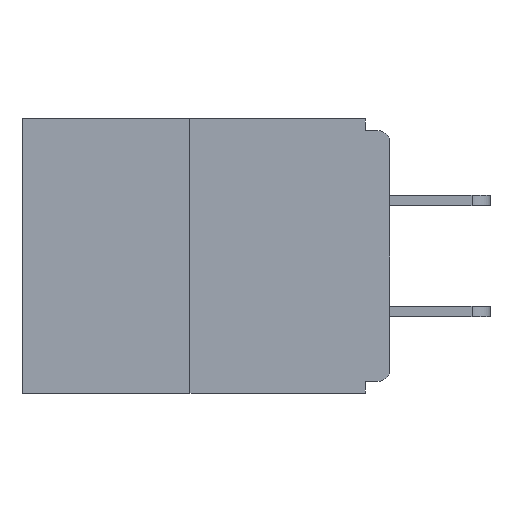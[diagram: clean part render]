
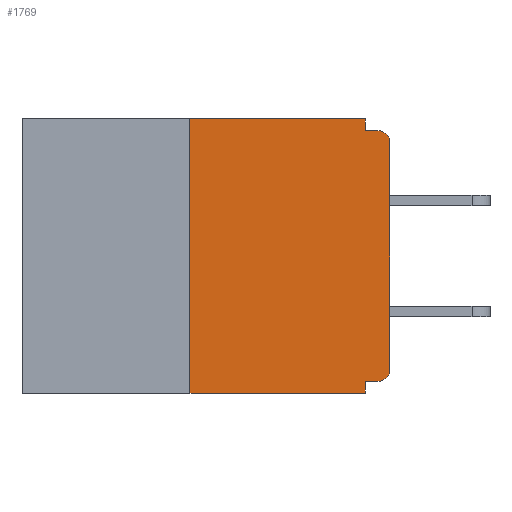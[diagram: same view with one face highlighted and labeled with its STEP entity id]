
A CAD part, left-side view. The second image highlights one B-rep face of the part: STEP entity #1769.
In plain terms, the highlighted planar face has unit normal (-1, 0, 0).
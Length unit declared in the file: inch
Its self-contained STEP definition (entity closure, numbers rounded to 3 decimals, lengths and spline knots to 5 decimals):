
#160 = DIRECTION ( 'NONE',  ( 0., 0., 1. ) ) ;
#436 = VECTOR ( 'NONE', #3665, 39.37008 ) ;
#724 = LINE ( 'NONE', #1875, #4259 ) ;
#869 = AXIS2_PLACEMENT_3D ( 'NONE', #11613, #14555, #8751 ) ;
#894 = CARTESIAN_POINT ( 'NONE',  ( 0., 0.031, 0. ) ) ;
#1299 = ORIENTED_EDGE ( 'NONE', *, *, #5207, .T. ) ;
#1614 = ORIENTED_EDGE ( 'NONE', *, *, #3676, .F. ) ;
#1615 = AXIS2_PLACEMENT_3D ( 'NONE', #4529, #18069, #1640 ) ;
#1617 = VERTEX_POINT ( 'NONE', #5138 ) ;
#1640 = DIRECTION ( 'NONE',  ( 0., 0., -1. ) ) ;
#1769 = ADVANCED_FACE ( 'NONE', ( #7443 ), #2712, .F. ) ;
#1875 = CARTESIAN_POINT ( 'NONE',  ( 0., 0., -0.328 ) ) ;
#1895 = CARTESIAN_POINT ( 'NONE',  ( 0., 0.25, 0. ) ) ;
#1930 = DIRECTION ( 'NONE',  ( 0., 0., -1. ) ) ;
#2110 = CIRCLE ( 'NONE', #1615, 0.015 ) ;
#2246 = LINE ( 'NONE', #9759, #15585 ) ;
#2348 = CARTESIAN_POINT ( 'NONE',  ( 0., 0.25, 0. ) ) ;
#2377 = VERTEX_POINT ( 'NONE', #2348 ) ;
#2414 = VERTEX_POINT ( 'NONE', #13216 ) ;
#2545 = CARTESIAN_POINT ( 'NONE',  ( 0., 0.031, -0.015 ) ) ;
#2712 = PLANE ( 'NONE',  #869 ) ;
#2959 = EDGE_CURVE ( 'NONE', #11232, #11114, #17690, .T. ) ;
#3665 = DIRECTION ( 'NONE',  ( 0., -1., 0. ) ) ;
#3676 = EDGE_CURVE ( 'NONE', #7419, #2377, #12792, .T. ) ;
#3739 = EDGE_CURVE ( 'NONE', #3911, #11114, #2246, .T. ) ;
#3911 = VERTEX_POINT ( 'NONE', #2545 ) ;
#4155 = AXIS2_PLACEMENT_3D ( 'NONE', #6329, #9402, #1930 ) ;
#4259 = VECTOR ( 'NONE', #15432, 39.37008 ) ;
#4289 = CARTESIAN_POINT ( 'NONE',  ( 0., 0.031, -0.343 ) ) ;
#4529 = CARTESIAN_POINT ( 'NONE',  ( 0., 0.015, -0.313 ) ) ;
#4957 = LINE ( 'NONE', #18576, #6845 ) ;
#5138 = CARTESIAN_POINT ( 'NONE',  ( 0., 0.031, -0.343 ) ) ;
#5207 = EDGE_CURVE ( 'NONE', #8612, #11232, #4957, .T. ) ;
#5284 = CARTESIAN_POINT ( 'NONE',  ( 0., 0.031, 0. ) ) ;
#5716 = CARTESIAN_POINT ( 'NONE',  ( 0., 0., -0.03 ) ) ;
#5815 = LINE ( 'NONE', #13789, #17277 ) ;
#6329 = CARTESIAN_POINT ( 'NONE',  ( 0., 0.015, -0.03 ) ) ;
#6691 = VERTEX_POINT ( 'NONE', #16149 ) ;
#6802 = LINE ( 'NONE', #10971, #436 ) ;
#6845 = VECTOR ( 'NONE', #160, 39.37008 ) ;
#7037 = ORIENTED_EDGE ( 'NONE', *, *, #9891, .F. ) ;
#7262 = EDGE_CURVE ( 'NONE', #7419, #1617, #5815, .T. ) ;
#7419 = VERTEX_POINT ( 'NONE', #10293 ) ;
#7443 = FACE_OUTER_BOUND ( 'NONE', #12723, .T. ) ;
#8161 = VECTOR ( 'NONE', #15756, 39.37008 ) ;
#8374 = ORIENTED_EDGE ( 'NONE', *, *, #7262, .T. ) ;
#8612 = VERTEX_POINT ( 'NONE', #14060 ) ;
#8751 = DIRECTION ( 'NONE',  ( 0., 0., -1. ) ) ;
#8767 = ORIENTED_EDGE ( 'NONE', *, *, #17659, .T. ) ;
#9286 = VECTOR ( 'NONE', #16694, 39.37008 ) ;
#9402 = DIRECTION ( 'NONE',  ( -1., 0., 0. ) ) ;
#9759 = CARTESIAN_POINT ( 'NONE',  ( 0., 0., -0.015 ) ) ;
#9891 = EDGE_CURVE ( 'NONE', #2414, #6691, #724, .T. ) ;
#10144 = ORIENTED_EDGE ( 'NONE', *, *, #3739, .F. ) ;
#10293 = CARTESIAN_POINT ( 'NONE',  ( 0., 0.25, -0.343 ) ) ;
#10938 = EDGE_CURVE ( 'NONE', #6691, #1617, #17651, .T. ) ;
#10971 = CARTESIAN_POINT ( 'NONE',  ( 0., 0.46, 0. ) ) ;
#11114 = VERTEX_POINT ( 'NONE', #13187 ) ;
#11232 = VERTEX_POINT ( 'NONE', #5716 ) ;
#11613 = CARTESIAN_POINT ( 'NONE',  ( 0., 0.46, 0. ) ) ;
#11890 = LINE ( 'NONE', #5284, #8161 ) ;
#12584 = ORIENTED_EDGE ( 'NONE', *, *, #10938, .F. ) ;
#12723 = EDGE_LOOP ( 'NONE', ( #19132, #1614, #8374, #12584, #7037, #8767, #1299, #17927, #10144, #18268 ) ) ;
#12772 = DIRECTION ( 'NONE',  ( 0., -1., 0. ) ) ;
#12792 = LINE ( 'NONE', #1895, #9286 ) ;
#13187 = CARTESIAN_POINT ( 'NONE',  ( 0., 0.015, -0.015 ) ) ;
#13216 = CARTESIAN_POINT ( 'NONE',  ( 0., 0.015, -0.328 ) ) ;
#13696 = VECTOR ( 'NONE', #16286, 39.37008 ) ;
#13789 = CARTESIAN_POINT ( 'NONE',  ( 0., 0.46, -0.343 ) ) ;
#13877 = EDGE_CURVE ( 'NONE', #2377, #16123, #6802, .T. ) ;
#14060 = CARTESIAN_POINT ( 'NONE',  ( 0., 0., -0.313 ) ) ;
#14555 = DIRECTION ( 'NONE',  ( 1., 0., 0. ) ) ;
#15273 = EDGE_CURVE ( 'NONE', #16123, #3911, #11890, .T. ) ;
#15432 = DIRECTION ( 'NONE',  ( 0., 1., 0. ) ) ;
#15585 = VECTOR ( 'NONE', #12772, 39.37008 ) ;
#15756 = DIRECTION ( 'NONE',  ( 0., 0., -1. ) ) ;
#16123 = VERTEX_POINT ( 'NONE', #894 ) ;
#16149 = CARTESIAN_POINT ( 'NONE',  ( 0., 0.031, -0.328 ) ) ;
#16286 = DIRECTION ( 'NONE',  ( 0., 0., -1. ) ) ;
#16694 = DIRECTION ( 'NONE',  ( 0., 0., 1. ) ) ;
#17044 = DIRECTION ( 'NONE',  ( 0., -1., 0. ) ) ;
#17277 = VECTOR ( 'NONE', #17044, 39.37008 ) ;
#17651 = LINE ( 'NONE', #4289, #13696 ) ;
#17659 = EDGE_CURVE ( 'NONE', #2414, #8612, #2110, .T. ) ;
#17690 = CIRCLE ( 'NONE', #4155, 0.015 ) ;
#17927 = ORIENTED_EDGE ( 'NONE', *, *, #2959, .T. ) ;
#18069 = DIRECTION ( 'NONE',  ( -1., 0., 0. ) ) ;
#18268 = ORIENTED_EDGE ( 'NONE', *, *, #15273, .F. ) ;
#18576 = CARTESIAN_POINT ( 'NONE',  ( 0., 0., 0. ) ) ;
#19132 = ORIENTED_EDGE ( 'NONE', *, *, #13877, .F. ) ;
